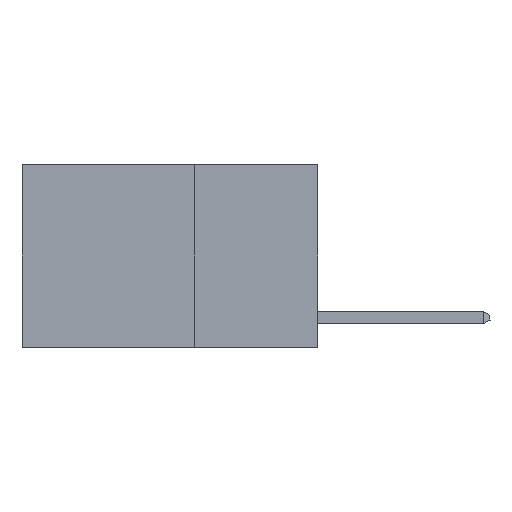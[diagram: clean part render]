
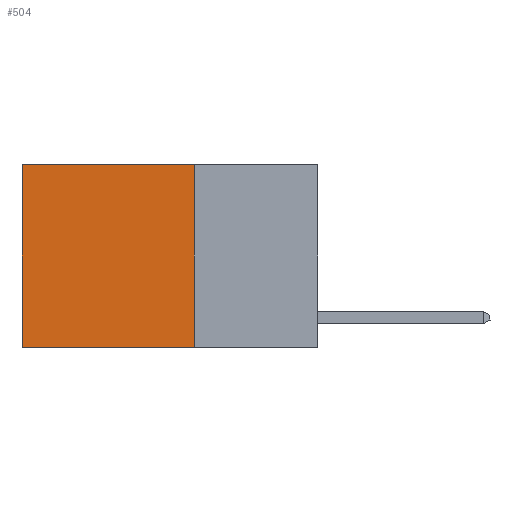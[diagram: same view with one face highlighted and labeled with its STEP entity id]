
A CAD part, left-side view. The second image highlights one B-rep face of the part: STEP entity #504.
In plain terms, the highlighted planar face has unit normal (-1, 0, 0).
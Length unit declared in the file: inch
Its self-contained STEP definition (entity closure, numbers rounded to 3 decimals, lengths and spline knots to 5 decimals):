
#218 = AXIS2_PLACEMENT_3D ( 'NONE', #13426, #15498, #3011 ) ;
#398 = VERTEX_POINT ( 'NONE', #25525 ) ;
#504 = ADVANCED_FACE ( 'NONE', ( #25964 ), #15410, .F. ) ;
#537 = DIRECTION ( 'NONE',  ( 0., 1., 0. ) ) ;
#1311 = CARTESIAN_POINT ( 'NONE',  ( 0.2625, 0.25, 0. ) ) ;
#1732 = ORIENTED_EDGE ( 'NONE', *, *, #11692, .F. ) ;
#3011 = DIRECTION ( 'NONE',  ( 0., 0., -1. ) ) ;
#4366 = VERTEX_POINT ( 'NONE', #1311 ) ;
#4436 = LINE ( 'NONE', #19244, #8694 ) ;
#6642 = CARTESIAN_POINT ( 'NONE',  ( 0.2625, 0.6, 0. ) ) ;
#7173 = DIRECTION ( 'NONE',  ( 0., 1., 0. ) ) ;
#8694 = VECTOR ( 'NONE', #537, 39.37008 ) ;
#8963 = VERTEX_POINT ( 'NONE', #21495 ) ;
#9001 = LINE ( 'NONE', #9177, #24919 ) ;
#9177 = CARTESIAN_POINT ( 'NONE',  ( 0.2625, 0.25, 0. ) ) ;
#9348 = CARTESIAN_POINT ( 'NONE',  ( 0.2625, 0.25, -0.37 ) ) ;
#10372 = ORIENTED_EDGE ( 'NONE', *, *, #20029, .T. ) ;
#10378 = VERTEX_POINT ( 'NONE', #9348 ) ;
#11313 = VECTOR ( 'NONE', #11624, 39.37008 ) ;
#11624 = DIRECTION ( 'NONE',  ( 0., 0., -1. ) ) ;
#11692 = EDGE_CURVE ( 'NONE', #4366, #10378, #16837, .T. ) ;
#11768 = LINE ( 'NONE', #6642, #16634 ) ;
#13253 = ORIENTED_EDGE ( 'NONE', *, *, #24423, .T. ) ;
#13426 = CARTESIAN_POINT ( 'NONE',  ( 0.2625, 0.25, 0. ) ) ;
#15410 = PLANE ( 'NONE',  #218 ) ;
#15498 = DIRECTION ( 'NONE',  ( 1., 0., 0. ) ) ;
#16002 = EDGE_CURVE ( 'NONE', #10378, #398, #4436, .T. ) ;
#16634 = VECTOR ( 'NONE', #21245, 39.37008 ) ;
#16837 = LINE ( 'NONE', #24053, #11313 ) ;
#18941 = EDGE_LOOP ( 'NONE', ( #10372, #22118, #1732, #13253 ) ) ;
#19244 = CARTESIAN_POINT ( 'NONE',  ( 0.2625, 0.25, -0.37 ) ) ;
#20029 = EDGE_CURVE ( 'NONE', #8963, #398, #11768, .T. ) ;
#21245 = DIRECTION ( 'NONE',  ( 0., 0., -1. ) ) ;
#21495 = CARTESIAN_POINT ( 'NONE',  ( 0.2625, 0.6, 0. ) ) ;
#22118 = ORIENTED_EDGE ( 'NONE', *, *, #16002, .F. ) ;
#24053 = CARTESIAN_POINT ( 'NONE',  ( 0.2625, 0.25, 0. ) ) ;
#24423 = EDGE_CURVE ( 'NONE', #4366, #8963, #9001, .T. ) ;
#24919 = VECTOR ( 'NONE', #7173, 39.37008 ) ;
#25525 = CARTESIAN_POINT ( 'NONE',  ( 0.2625, 0.6, -0.37 ) ) ;
#25964 = FACE_OUTER_BOUND ( 'NONE', #18941, .T. ) ;
